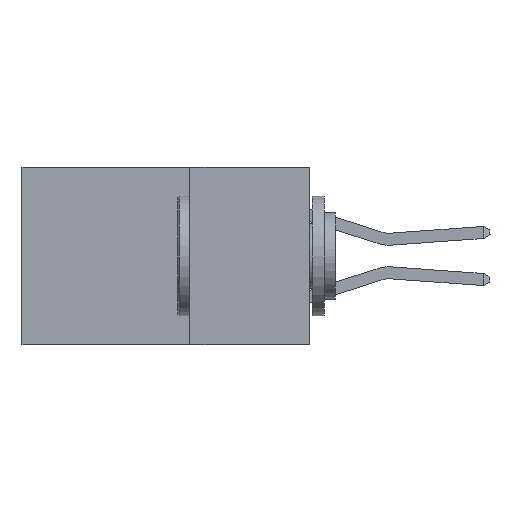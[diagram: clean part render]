
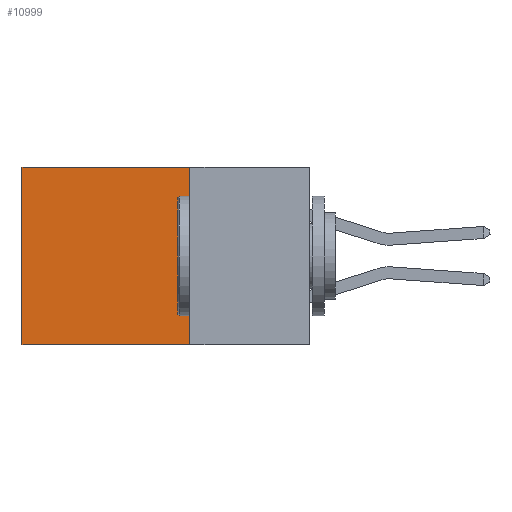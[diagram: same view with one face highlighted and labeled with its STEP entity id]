
A CAD part, left-side view. The second image highlights one B-rep face of the part: STEP entity #10999.
In plain terms, the highlighted planar face has unit normal (-1, 0, 0).
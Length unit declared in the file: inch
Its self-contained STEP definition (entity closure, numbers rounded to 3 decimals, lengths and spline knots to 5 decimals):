
#45 = CARTESIAN_POINT ( 'NONE',  ( 0.2615, 0.25, -0.37 ) ) ;
#379 = LINE ( 'NONE', #9524, #9474 ) ;
#432 = CARTESIAN_POINT ( 'NONE',  ( 0.2615, 0.6, 0. ) ) ;
#575 = FACE_OUTER_BOUND ( 'NONE', #7667, .T. ) ;
#986 = DIRECTION ( 'NONE',  ( 0., 0., -1. ) ) ;
#1088 = CARTESIAN_POINT ( 'NONE',  ( 0.2615, 0.25, 0. ) ) ;
#1110 = CARTESIAN_POINT ( 'NONE',  ( 0.2615, 0.25, -0.37 ) ) ;
#1180 = LINE ( 'NONE', #1110, #7252 ) ;
#1240 = DIRECTION ( 'NONE',  ( 0., 0., -1. ) ) ;
#1421 = EDGE_CURVE ( 'NONE', #9986, #8119, #379, .T. ) ;
#2129 = ORIENTED_EDGE ( 'NONE', *, *, #1421, .T. ) ;
#2354 = LINE ( 'NONE', #3959, #6336 ) ;
#3414 = AXIS2_PLACEMENT_3D ( 'NONE', #45, #6089, #986 ) ;
#3799 = VERTEX_POINT ( 'NONE', #5567 ) ;
#3918 = DIRECTION ( 'NONE',  ( 0., 1., 0. ) ) ;
#3959 = CARTESIAN_POINT ( 'NONE',  ( 0.2615, 0.25, -0.37 ) ) ;
#4102 = EDGE_CURVE ( 'NONE', #9986, #5292, #1180, .T. ) ;
#4343 = PLANE ( 'NONE',  #3414 ) ;
#4521 = DIRECTION ( 'NONE',  ( 0., 0., -1. ) ) ;
#4696 = CARTESIAN_POINT ( 'NONE',  ( 0.2615, 0.6, -0.37 ) ) ;
#5080 = VECTOR ( 'NONE', #4521, 39.37008 ) ;
#5292 = VERTEX_POINT ( 'NONE', #7955 ) ;
#5298 = ORIENTED_EDGE ( 'NONE', *, *, #5750, .F. ) ;
#5567 = CARTESIAN_POINT ( 'NONE',  ( 0.2615, 0.6, -0.37 ) ) ;
#5661 = EDGE_CURVE ( 'NONE', #8119, #3799, #7805, .T. ) ;
#5750 = EDGE_CURVE ( 'NONE', #5292, #3799, #2354, .T. ) ;
#6089 = DIRECTION ( 'NONE',  ( 1., 0., 0. ) ) ;
#6336 = VECTOR ( 'NONE', #3918, 39.37008 ) ;
#6355 = ORIENTED_EDGE ( 'NONE', *, *, #4102, .F. ) ;
#7252 = VECTOR ( 'NONE', #1240, 39.37008 ) ;
#7667 = EDGE_LOOP ( 'NONE', ( #9806, #5298, #6355, #2129 ) ) ;
#7805 = LINE ( 'NONE', #4696, #5080 ) ;
#7955 = CARTESIAN_POINT ( 'NONE',  ( 0.2615, 0.25, -0.37 ) ) ;
#8119 = VERTEX_POINT ( 'NONE', #432 ) ;
#9474 = VECTOR ( 'NONE', #9812, 39.37008 ) ;
#9524 = CARTESIAN_POINT ( 'NONE',  ( 0.2615, 0.25, 0. ) ) ;
#9806 = ORIENTED_EDGE ( 'NONE', *, *, #5661, .T. ) ;
#9812 = DIRECTION ( 'NONE',  ( 0., 1., 0. ) ) ;
#9986 = VERTEX_POINT ( 'NONE', #1088 ) ;
#10999 = ADVANCED_FACE ( 'NONE', ( #575 ), #4343, .F. ) ;
